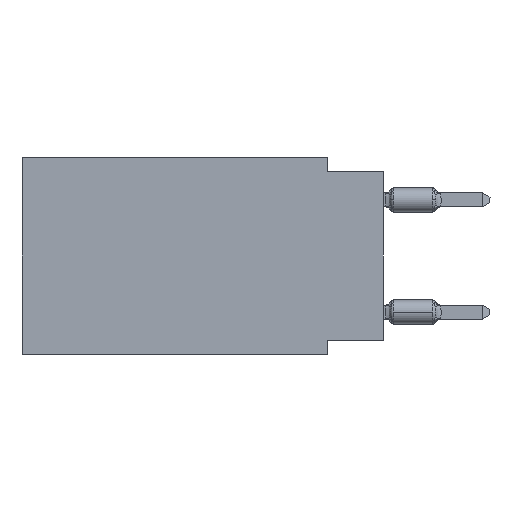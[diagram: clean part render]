
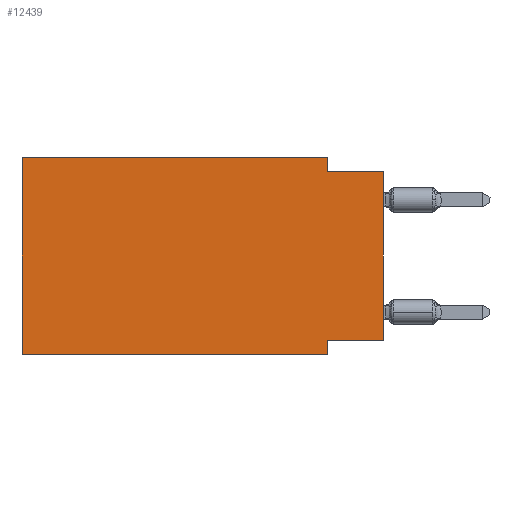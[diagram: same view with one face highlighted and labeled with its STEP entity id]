
A CAD part, left-side view. The second image highlights one B-rep face of the part: STEP entity #12439.
In plain terms, the highlighted planar face has unit normal (-1, 0, 0).
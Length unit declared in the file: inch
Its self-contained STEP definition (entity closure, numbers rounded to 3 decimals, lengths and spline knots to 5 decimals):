
#19 = ORIENTED_EDGE ( 'NONE', *, *, #10482, .F. ) ;
#22 = ORIENTED_EDGE ( 'NONE', *, *, #9342, .T. ) ;
#153 = ORIENTED_EDGE ( 'NONE', *, *, #11538, .F. ) ;
#1357 = DIRECTION ( 'NONE',  ( 0., 1., 0. ) ) ;
#1361 = LINE ( 'NONE', #11993, #7261 ) ;
#1446 = DIRECTION ( 'NONE',  ( 0., -1., 0. ) ) ;
#2206 = CARTESIAN_POINT ( 'NONE',  ( 0., 0.645, 0. ) ) ;
#2333 = CARTESIAN_POINT ( 'NONE',  ( 0., 0.1, 0. ) ) ;
#2347 = CARTESIAN_POINT ( 'NONE',  ( 0., 0.1, -0.325 ) ) ;
#2757 = VERTEX_POINT ( 'NONE', #3907 ) ;
#3101 = EDGE_CURVE ( 'NONE', #12039, #10743, #1361, .T. ) ;
#3907 = CARTESIAN_POINT ( 'NONE',  ( 0., 0.1, -0.35 ) ) ;
#4050 = DIRECTION ( 'NONE',  ( 0., 0., 1. ) ) ;
#4107 = LINE ( 'NONE', #13443, #13842 ) ;
#4410 = LINE ( 'NONE', #4556, #14067 ) ;
#4556 = CARTESIAN_POINT ( 'NONE',  ( 0., 0.645, 0. ) ) ;
#4655 = LINE ( 'NONE', #5511, #8548 ) ;
#4715 = AXIS2_PLACEMENT_3D ( 'NONE', #13330, #5071, #14480 ) ;
#5043 = VERTEX_POINT ( 'NONE', #2347 ) ;
#5053 = LINE ( 'NONE', #9627, #9699 ) ;
#5070 = EDGE_CURVE ( 'NONE', #5043, #2757, #4655, .T. ) ;
#5071 = DIRECTION ( 'NONE',  ( 1., 0., 0. ) ) ;
#5108 = DIRECTION ( 'NONE',  ( 0., 0., 1. ) ) ;
#5376 = PLANE ( 'NONE',  #4715 ) ;
#5511 = CARTESIAN_POINT ( 'NONE',  ( 0., 0.1, -0.35 ) ) ;
#6824 = CARTESIAN_POINT ( 'NONE',  ( 0., 0., -0.325 ) ) ;
#6980 = DIRECTION ( 'NONE',  ( 0., -1., 0. ) ) ;
#7109 = ORIENTED_EDGE ( 'NONE', *, *, #3101, .F. ) ;
#7199 = CARTESIAN_POINT ( 'NONE',  ( 0., 0., -0.325 ) ) ;
#7261 = VECTOR ( 'NONE', #6980, 39.37008 ) ;
#7783 = CARTESIAN_POINT ( 'NONE',  ( 0., 0., -0.025 ) ) ;
#8119 = ORIENTED_EDGE ( 'NONE', *, *, #13156, .F. ) ;
#8175 = VERTEX_POINT ( 'NONE', #9852 ) ;
#8480 = VECTOR ( 'NONE', #8669, 39.37008 ) ;
#8531 = LINE ( 'NONE', #13307, #13858 ) ;
#8548 = VECTOR ( 'NONE', #10235, 39.37008 ) ;
#8627 = FACE_OUTER_BOUND ( 'NONE', #13635, .T. ) ;
#8669 = DIRECTION ( 'NONE',  ( 0., 0., -1. ) ) ;
#8679 = VECTOR ( 'NONE', #1357, 39.37008 ) ;
#9342 = EDGE_CURVE ( 'NONE', #8175, #2757, #5053, .T. ) ;
#9627 = CARTESIAN_POINT ( 'NONE',  ( 0., 0.645, -0.35 ) ) ;
#9680 = VERTEX_POINT ( 'NONE', #6824 ) ;
#9699 = VECTOR ( 'NONE', #1446, 39.37008 ) ;
#9852 = CARTESIAN_POINT ( 'NONE',  ( 0., 0.645, -0.35 ) ) ;
#10235 = DIRECTION ( 'NONE',  ( 0., 0., -1. ) ) ;
#10482 = EDGE_CURVE ( 'NONE', #14183, #13454, #4410, .T. ) ;
#10509 = DIRECTION ( 'NONE',  ( 0., -1., 0. ) ) ;
#10743 = VERTEX_POINT ( 'NONE', #7783 ) ;
#10931 = CARTESIAN_POINT ( 'NONE',  ( 0., 0.1, 0. ) ) ;
#11538 = EDGE_CURVE ( 'NONE', #8175, #14183, #8531, .T. ) ;
#11993 = CARTESIAN_POINT ( 'NONE',  ( 0., 0., -0.025 ) ) ;
#12039 = VERTEX_POINT ( 'NONE', #13658 ) ;
#12154 = ORIENTED_EDGE ( 'NONE', *, *, #5070, .F. ) ;
#12439 = ADVANCED_FACE ( 'NONE', ( #8627 ), #5376, .F. ) ;
#12833 = ORIENTED_EDGE ( 'NONE', *, *, #13189, .T. ) ;
#13156 = EDGE_CURVE ( 'NONE', #9680, #5043, #14213, .T. ) ;
#13189 = EDGE_CURVE ( 'NONE', #9680, #10743, #4107, .T. ) ;
#13307 = CARTESIAN_POINT ( 'NONE',  ( 0., 0.645, 0. ) ) ;
#13330 = CARTESIAN_POINT ( 'NONE',  ( 0., 0.645, 0. ) ) ;
#13443 = CARTESIAN_POINT ( 'NONE',  ( 0., 0., 0. ) ) ;
#13454 = VERTEX_POINT ( 'NONE', #2333 ) ;
#13635 = EDGE_LOOP ( 'NONE', ( #12833, #7109, #13742, #19, #153, #22, #12154, #8119 ) ) ;
#13658 = CARTESIAN_POINT ( 'NONE',  ( 0., 0.1, -0.025 ) ) ;
#13742 = ORIENTED_EDGE ( 'NONE', *, *, #14447, .F. ) ;
#13842 = VECTOR ( 'NONE', #5108, 39.37008 ) ;
#13858 = VECTOR ( 'NONE', #4050, 39.37008 ) ;
#14067 = VECTOR ( 'NONE', #10509, 39.37008 ) ;
#14183 = VERTEX_POINT ( 'NONE', #2206 ) ;
#14213 = LINE ( 'NONE', #7199, #8679 ) ;
#14295 = LINE ( 'NONE', #10931, #8480 ) ;
#14447 = EDGE_CURVE ( 'NONE', #13454, #12039, #14295, .T. ) ;
#14480 = DIRECTION ( 'NONE',  ( 0., 0., -1. ) ) ;
